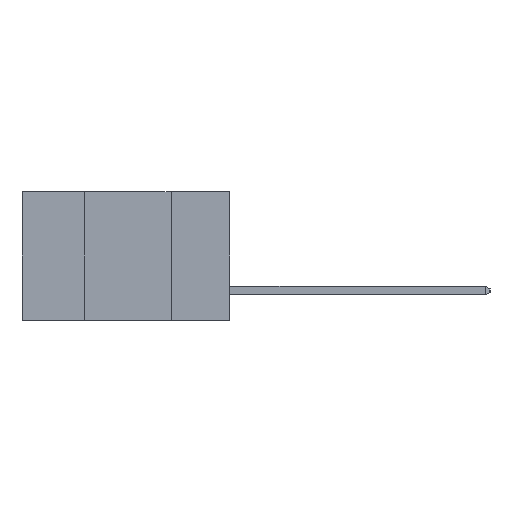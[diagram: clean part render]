
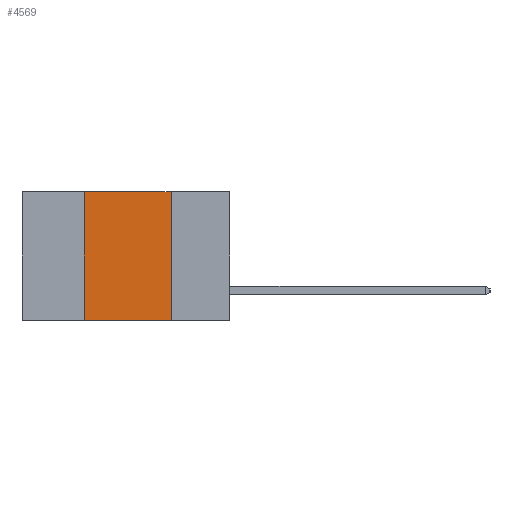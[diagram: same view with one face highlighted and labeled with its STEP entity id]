
A CAD part, left-side view. The second image highlights one B-rep face of the part: STEP entity #4569.
In plain terms, the highlighted planar face has unit normal (-1, 0, 0).
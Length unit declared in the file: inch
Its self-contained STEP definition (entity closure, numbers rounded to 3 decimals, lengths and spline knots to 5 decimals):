
#34 = LINE ( 'NONE', #3744, #8084 ) ;
#43 = EDGE_LOOP ( 'NONE', ( #1846, #3379, #6140, #4231 ) ) ;
#282 = EDGE_CURVE ( 'NONE', #1292, #11470, #34, .T. ) ;
#696 = AXIS2_PLACEMENT_3D ( 'NONE', #6009, #9545, #2272 ) ;
#988 = CARTESIAN_POINT ( 'NONE',  ( 0., 0.17, -0.37 ) ) ;
#1292 = VERTEX_POINT ( 'NONE', #5891 ) ;
#1637 = LINE ( 'NONE', #4807, #6880 ) ;
#1846 = ORIENTED_EDGE ( 'NONE', *, *, #282, .F. ) ;
#2272 = DIRECTION ( 'NONE',  ( 0., 0., -1. ) ) ;
#2703 = VECTOR ( 'NONE', #6026, 39.37008 ) ;
#3042 = LINE ( 'NONE', #9099, #2703 ) ;
#3379 = ORIENTED_EDGE ( 'NONE', *, *, #6800, .F. ) ;
#3692 = FACE_OUTER_BOUND ( 'NONE', #43, .T. ) ;
#3744 = CARTESIAN_POINT ( 'NONE',  ( 0., 0.17, 0. ) ) ;
#4231 = ORIENTED_EDGE ( 'NONE', *, *, #10971, .T. ) ;
#4569 = ADVANCED_FACE ( 'NONE', ( #3692 ), #11557, .F. ) ;
#4807 = CARTESIAN_POINT ( 'NONE',  ( 0., 0.6, 0. ) ) ;
#5129 = LINE ( 'NONE', #12622, #12583 ) ;
#5826 = DIRECTION ( 'NONE',  ( 0., -1., 0. ) ) ;
#5891 = CARTESIAN_POINT ( 'NONE',  ( 0., 0.17, 0. ) ) ;
#6009 = CARTESIAN_POINT ( 'NONE',  ( 0., 0.6, 0. ) ) ;
#6026 = DIRECTION ( 'NONE',  ( 0., 0., 1. ) ) ;
#6140 = ORIENTED_EDGE ( 'NONE', *, *, #12967, .F. ) ;
#6558 = DIRECTION ( 'NONE',  ( 0., -1., 0. ) ) ;
#6683 = DIRECTION ( 'NONE',  ( 0., 0., -1. ) ) ;
#6800 = EDGE_CURVE ( 'NONE', #10346, #1292, #1637, .T. ) ;
#6880 = VECTOR ( 'NONE', #5826, 39.37008 ) ;
#8084 = VECTOR ( 'NONE', #6683, 39.37008 ) ;
#8248 = CARTESIAN_POINT ( 'NONE',  ( 0., 0.42, -0.37 ) ) ;
#9099 = CARTESIAN_POINT ( 'NONE',  ( 0., 0.42, 0. ) ) ;
#9545 = DIRECTION ( 'NONE',  ( 1., 0., 0. ) ) ;
#10346 = VERTEX_POINT ( 'NONE', #12683 ) ;
#10971 = EDGE_CURVE ( 'NONE', #12038, #11470, #5129, .T. ) ;
#11470 = VERTEX_POINT ( 'NONE', #988 ) ;
#11557 = PLANE ( 'NONE',  #696 ) ;
#12038 = VERTEX_POINT ( 'NONE', #8248 ) ;
#12583 = VECTOR ( 'NONE', #6558, 39.37008 ) ;
#12622 = CARTESIAN_POINT ( 'NONE',  ( 0., 0.6, -0.37 ) ) ;
#12683 = CARTESIAN_POINT ( 'NONE',  ( 0., 0.42, 0. ) ) ;
#12967 = EDGE_CURVE ( 'NONE', #12038, #10346, #3042, .T. ) ;
